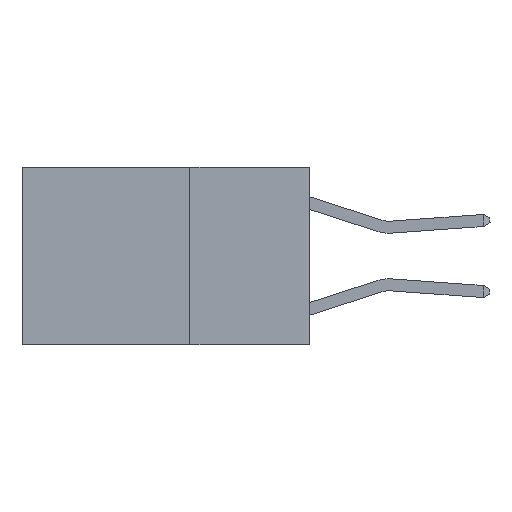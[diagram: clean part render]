
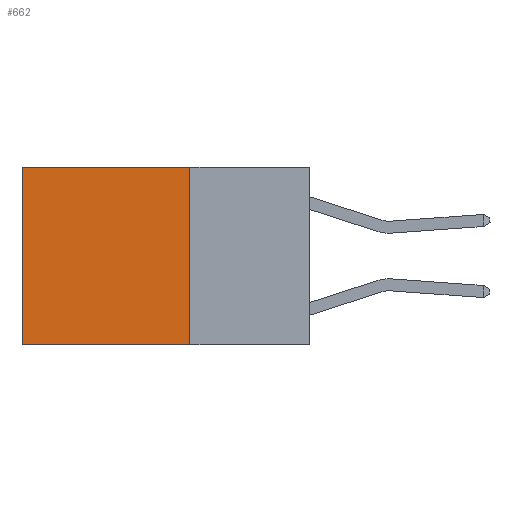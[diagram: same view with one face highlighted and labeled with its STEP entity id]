
A CAD part, left-side view. The second image highlights one B-rep face of the part: STEP entity #662.
In plain terms, the highlighted planar face has unit normal (-1, 0, 0).
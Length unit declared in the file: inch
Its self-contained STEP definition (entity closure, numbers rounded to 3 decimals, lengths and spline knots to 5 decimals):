
#94 = VECTOR ( 'NONE', #11289, 39.37008 ) ;
#241 = DIRECTION ( 'NONE',  ( 1., 0., 0. ) ) ;
#662 = ADVANCED_FACE ( 'NONE', ( #10383 ), #1799, .F. ) ;
#1179 = VECTOR ( 'NONE', #8231, 39.37008 ) ;
#1428 = ORIENTED_EDGE ( 'NONE', *, *, #5236, .T. ) ;
#1488 = LINE ( 'NONE', #10176, #1179 ) ;
#1578 = DIRECTION ( 'NONE',  ( 0., 1., 0. ) ) ;
#1608 = CARTESIAN_POINT ( 'NONE',  ( 0.2625, 0.25, 0. ) ) ;
#1799 = PLANE ( 'NONE',  #4818 ) ;
#2243 = VERTEX_POINT ( 'NONE', #3964 ) ;
#2612 = CARTESIAN_POINT ( 'NONE',  ( 0.2625, 0.25, 0. ) ) ;
#2965 = LINE ( 'NONE', #5843, #5389 ) ;
#3685 = CARTESIAN_POINT ( 'NONE',  ( 0.2625, 0.6, -0.37 ) ) ;
#3964 = CARTESIAN_POINT ( 'NONE',  ( 0.2625, 0.6, 0. ) ) ;
#4818 = AXIS2_PLACEMENT_3D ( 'NONE', #2612, #241, #7951 ) ;
#5236 = EDGE_CURVE ( 'NONE', #8022, #2243, #12396, .T. ) ;
#5316 = CARTESIAN_POINT ( 'NONE',  ( 0.2625, 0.6, 0. ) ) ;
#5389 = VECTOR ( 'NONE', #10864, 39.37008 ) ;
#5843 = CARTESIAN_POINT ( 'NONE',  ( 0.2625, 0.25, 0. ) ) ;
#6277 = EDGE_CURVE ( 'NONE', #2243, #11249, #11120, .T. ) ;
#6348 = VERTEX_POINT ( 'NONE', #6397 ) ;
#6397 = CARTESIAN_POINT ( 'NONE',  ( 0.2625, 0.25, -0.37 ) ) ;
#6900 = EDGE_CURVE ( 'NONE', #6348, #11249, #1488, .T. ) ;
#7658 = CARTESIAN_POINT ( 'NONE',  ( 0.2625, 0.25, 0. ) ) ;
#7951 = DIRECTION ( 'NONE',  ( 0., 0., -1. ) ) ;
#8022 = VERTEX_POINT ( 'NONE', #1608 ) ;
#8060 = EDGE_LOOP ( 'NONE', ( #9903, #11930, #12272, #1428 ) ) ;
#8231 = DIRECTION ( 'NONE',  ( 0., 1., 0. ) ) ;
#9903 = ORIENTED_EDGE ( 'NONE', *, *, #6277, .T. ) ;
#10176 = CARTESIAN_POINT ( 'NONE',  ( 0.2625, 0.25, -0.37 ) ) ;
#10383 = FACE_OUTER_BOUND ( 'NONE', #8060, .T. ) ;
#10864 = DIRECTION ( 'NONE',  ( 0., 0., -1. ) ) ;
#11120 = LINE ( 'NONE', #5316, #94 ) ;
#11249 = VERTEX_POINT ( 'NONE', #3685 ) ;
#11289 = DIRECTION ( 'NONE',  ( 0., 0., -1. ) ) ;
#11930 = ORIENTED_EDGE ( 'NONE', *, *, #6900, .F. ) ;
#12073 = VECTOR ( 'NONE', #1578, 39.37008 ) ;
#12272 = ORIENTED_EDGE ( 'NONE', *, *, #12740, .F. ) ;
#12396 = LINE ( 'NONE', #7658, #12073 ) ;
#12740 = EDGE_CURVE ( 'NONE', #8022, #6348, #2965, .T. ) ;
